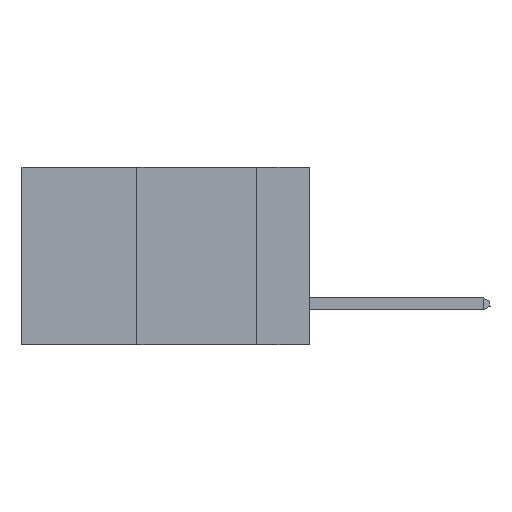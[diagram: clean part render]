
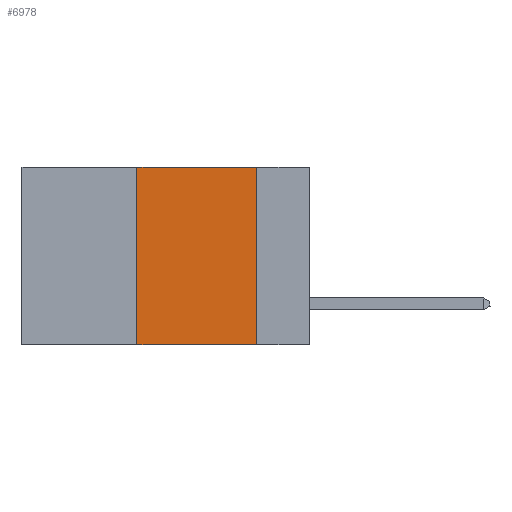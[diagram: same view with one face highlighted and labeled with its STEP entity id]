
A CAD part, left-side view. The second image highlights one B-rep face of the part: STEP entity #6978.
In plain terms, the highlighted planar face has unit normal (-1, 0, 0).
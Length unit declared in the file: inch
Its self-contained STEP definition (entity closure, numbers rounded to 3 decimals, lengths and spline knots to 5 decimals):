
#11 = DIRECTION ( 'NONE',  ( 1., 0., 0. ) ) ;
#591 = LINE ( 'NONE', #5894, #7835 ) ;
#732 = DIRECTION ( 'NONE',  ( 0., -1., 0. ) ) ;
#790 = AXIS2_PLACEMENT_3D ( 'NONE', #14506, #11, #10762 ) ;
#1244 = VERTEX_POINT ( 'NONE', #7496 ) ;
#1282 = ORIENTED_EDGE ( 'NONE', *, *, #10757, .T. ) ;
#1656 = ORIENTED_EDGE ( 'NONE', *, *, #11110, .F. ) ;
#2721 = LINE ( 'NONE', #9601, #4396 ) ;
#2829 = VERTEX_POINT ( 'NONE', #13042 ) ;
#3243 = VECTOR ( 'NONE', #4004, 39.37008 ) ;
#3502 = DIRECTION ( 'NONE',  ( 0., 0., -1. ) ) ;
#3504 = CARTESIAN_POINT ( 'NONE',  ( 0., 0.36, -0.37 ) ) ;
#4004 = DIRECTION ( 'NONE',  ( 0., -1., 0. ) ) ;
#4396 = VECTOR ( 'NONE', #3502, 39.37008 ) ;
#4672 = ORIENTED_EDGE ( 'NONE', *, *, #15445, .F. ) ;
#4890 = VECTOR ( 'NONE', #732, 39.37008 ) ;
#5173 = CARTESIAN_POINT ( 'NONE',  ( 0., 0.6, -0.37 ) ) ;
#5894 = CARTESIAN_POINT ( 'NONE',  ( 0., 0.36, 0. ) ) ;
#6760 = CARTESIAN_POINT ( 'NONE',  ( 0., 0.6, 0. ) ) ;
#6978 = ADVANCED_FACE ( 'NONE', ( #11158 ), #14410, .F. ) ;
#7496 = CARTESIAN_POINT ( 'NONE',  ( 0., 0.11, 0. ) ) ;
#7835 = VECTOR ( 'NONE', #9902, 39.37008 ) ;
#7952 = EDGE_LOOP ( 'NONE', ( #4672, #10514, #1656, #1282 ) ) ;
#9601 = CARTESIAN_POINT ( 'NONE',  ( 0., 0.11, 0. ) ) ;
#9902 = DIRECTION ( 'NONE',  ( 0., 0., 1. ) ) ;
#10514 = ORIENTED_EDGE ( 'NONE', *, *, #13591, .F. ) ;
#10757 = EDGE_CURVE ( 'NONE', #13713, #2829, #12740, .T. ) ;
#10762 = DIRECTION ( 'NONE',  ( 0., 0., -1. ) ) ;
#11110 = EDGE_CURVE ( 'NONE', #13713, #13923, #591, .T. ) ;
#11158 = FACE_OUTER_BOUND ( 'NONE', #7952, .T. ) ;
#11488 = LINE ( 'NONE', #6760, #4890 ) ;
#12740 = LINE ( 'NONE', #5173, #3243 ) ;
#13042 = CARTESIAN_POINT ( 'NONE',  ( 0., 0.11, -0.37 ) ) ;
#13591 = EDGE_CURVE ( 'NONE', #13923, #1244, #11488, .T. ) ;
#13713 = VERTEX_POINT ( 'NONE', #3504 ) ;
#13923 = VERTEX_POINT ( 'NONE', #14304 ) ;
#14304 = CARTESIAN_POINT ( 'NONE',  ( 0., 0.36, 0. ) ) ;
#14410 = PLANE ( 'NONE',  #790 ) ;
#14506 = CARTESIAN_POINT ( 'NONE',  ( 0., 0.6, 0. ) ) ;
#15445 = EDGE_CURVE ( 'NONE', #1244, #2829, #2721, .T. ) ;
